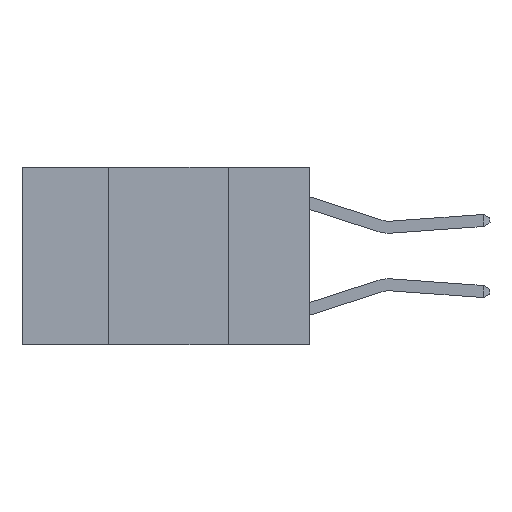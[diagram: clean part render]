
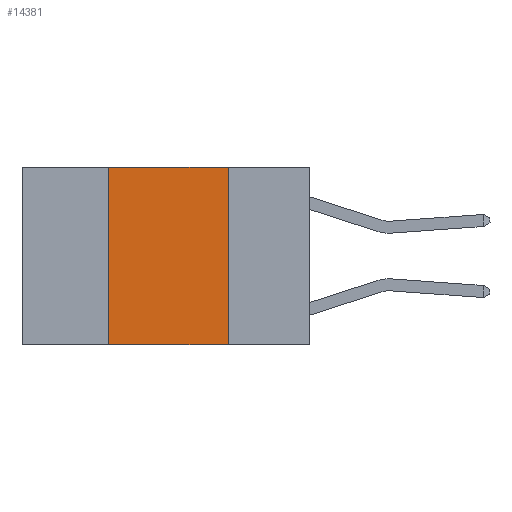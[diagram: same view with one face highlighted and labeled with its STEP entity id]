
A CAD part, left-side view. The second image highlights one B-rep face of the part: STEP entity #14381.
In plain terms, the highlighted planar face has unit normal (-1, 0, 0).
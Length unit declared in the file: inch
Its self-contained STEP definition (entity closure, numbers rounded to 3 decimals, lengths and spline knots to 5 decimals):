
#81 = ORIENTED_EDGE ( 'NONE', *, *, #8297, .F. ) ;
#455 = CARTESIAN_POINT ( 'NONE',  ( 0., 0.17, 0. ) ) ;
#632 = PLANE ( 'NONE',  #12440 ) ;
#736 = EDGE_CURVE ( 'NONE', #1041, #9657, #9957, .T. ) ;
#786 = CARTESIAN_POINT ( 'NONE',  ( 0., 0.42, 0. ) ) ;
#1041 = VERTEX_POINT ( 'NONE', #786 ) ;
#1415 = LINE ( 'NONE', #8930, #18522 ) ;
#3274 = DIRECTION ( 'NONE',  ( 0., 0., -1. ) ) ;
#4049 = DIRECTION ( 'NONE',  ( 1., 0., 0. ) ) ;
#4489 = EDGE_CURVE ( 'NONE', #17142, #1041, #19643, .T. ) ;
#4517 = ORIENTED_EDGE ( 'NONE', *, *, #736, .F. ) ;
#5694 = EDGE_LOOP ( 'NONE', ( #81, #4517, #9441, #18255 ) ) ;
#6483 = CARTESIAN_POINT ( 'NONE',  ( 0., 0.17, 0. ) ) ;
#7124 = VECTOR ( 'NONE', #3274, 39.37008 ) ;
#8120 = DIRECTION ( 'NONE',  ( 0., 0., 1. ) ) ;
#8297 = EDGE_CURVE ( 'NONE', #9657, #18176, #15949, .T. ) ;
#8930 = CARTESIAN_POINT ( 'NONE',  ( 0., 0.6, -0.37 ) ) ;
#9441 = ORIENTED_EDGE ( 'NONE', *, *, #4489, .F. ) ;
#9657 = VERTEX_POINT ( 'NONE', #455 ) ;
#9957 = LINE ( 'NONE', #21302, #18759 ) ;
#10178 = CARTESIAN_POINT ( 'NONE',  ( 0., 0.17, -0.37 ) ) ;
#12291 = DIRECTION ( 'NONE',  ( 0., -1., 0. ) ) ;
#12440 = AXIS2_PLACEMENT_3D ( 'NONE', #14007, #4049, #15687 ) ;
#13671 = EDGE_CURVE ( 'NONE', #17142, #18176, #1415, .T. ) ;
#14007 = CARTESIAN_POINT ( 'NONE',  ( 0., 0.6, 0. ) ) ;
#14381 = ADVANCED_FACE ( 'NONE', ( #17718 ), #632, .F. ) ;
#15312 = VECTOR ( 'NONE', #8120, 39.37008 ) ;
#15687 = DIRECTION ( 'NONE',  ( 0., 0., -1. ) ) ;
#15949 = LINE ( 'NONE', #6483, #7124 ) ;
#17142 = VERTEX_POINT ( 'NONE', #20813 ) ;
#17718 = FACE_OUTER_BOUND ( 'NONE', #5694, .T. ) ;
#18176 = VERTEX_POINT ( 'NONE', #10178 ) ;
#18255 = ORIENTED_EDGE ( 'NONE', *, *, #13671, .T. ) ;
#18522 = VECTOR ( 'NONE', #12291, 39.37008 ) ;
#18759 = VECTOR ( 'NONE', #20556, 39.37008 ) ;
#19643 = LINE ( 'NONE', #19652, #15312 ) ;
#19652 = CARTESIAN_POINT ( 'NONE',  ( 0., 0.42, 0. ) ) ;
#20556 = DIRECTION ( 'NONE',  ( 0., -1., 0. ) ) ;
#20813 = CARTESIAN_POINT ( 'NONE',  ( 0., 0.42, -0.37 ) ) ;
#21302 = CARTESIAN_POINT ( 'NONE',  ( 0., 0.6, 0. ) ) ;
